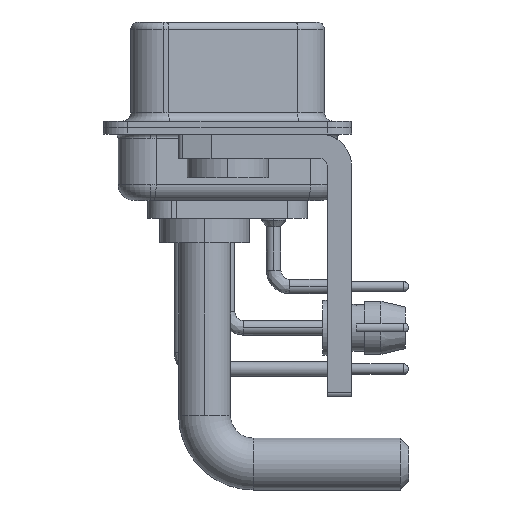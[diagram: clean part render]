
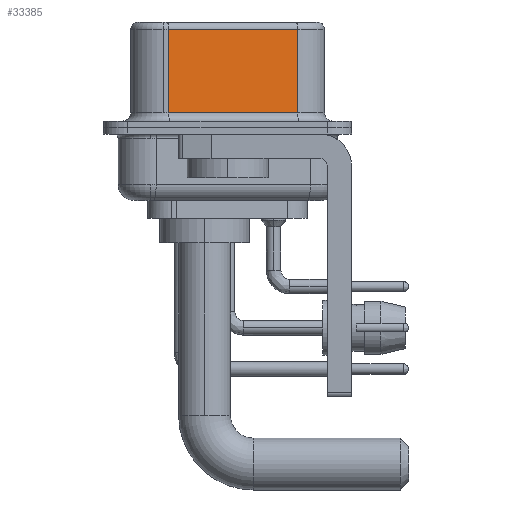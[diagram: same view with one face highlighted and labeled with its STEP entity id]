
A CAD part, left-side view. The second image highlights one B-rep face of the part: STEP entity #33385.
In plain terms, the highlighted planar face has unit normal (-0.985, -0.174, 0).
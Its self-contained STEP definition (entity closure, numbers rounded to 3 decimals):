
#1555 = CARTESIAN_POINT ( 'NONE',  ( 3.73, 3.628, 6.52 ) ) ;
#2030 = VECTOR ( 'NONE', #33905, 1000. ) ;
#3834 = VECTOR ( 'NONE', #34568, 1000. ) ;
#3892 = PLANE ( 'NONE',  #28740 ) ;
#5429 = VERTEX_POINT ( 'NONE', #19624 ) ;
#8009 = DIRECTION ( 'NONE',  ( -0.174, 0.985, 0. ) ) ;
#9073 = LINE ( 'NONE', #23927, #3834 ) ;
#9569 = CARTESIAN_POINT ( 'NONE',  ( 3.73, 3.628, 6.02 ) ) ;
#10023 = CARTESIAN_POINT ( 'NONE',  ( 5.132, -4.322, 6.52 ) ) ;
#13352 = EDGE_CURVE ( 'NONE', #21928, #5429, #9073, .T. ) ;
#14347 = LINE ( 'NONE', #24977, #2030 ) ;
#14448 = VERTEX_POINT ( 'NONE', #18462 ) ;
#14463 = VERTEX_POINT ( 'NONE', #9569 ) ;
#15104 = ORIENTED_EDGE ( 'NONE', *, *, #33988, .T. ) ;
#16024 = ORIENTED_EDGE ( 'NONE', *, *, #21166, .T. ) ;
#16779 = ORIENTED_EDGE ( 'NONE', *, *, #13352, .F. ) ;
#18462 = CARTESIAN_POINT ( 'NONE',  ( 3.73, 3.628, 0.9 ) ) ;
#19144 = LINE ( 'NONE', #33488, #27423 ) ;
#19624 = CARTESIAN_POINT ( 'NONE',  ( 5.132, -4.322, 0.9 ) ) ;
#21166 = EDGE_CURVE ( 'NONE', #21928, #14463, #19144, .T. ) ;
#21265 = LINE ( 'NONE', #1555, #33356 ) ;
#21466 = CARTESIAN_POINT ( 'NONE',  ( 5.132, -4.322, 6.02 ) ) ;
#21928 = VERTEX_POINT ( 'NONE', #21466 ) ;
#23927 = CARTESIAN_POINT ( 'NONE',  ( 5.132, -4.322, 6.52 ) ) ;
#24977 = CARTESIAN_POINT ( 'NONE',  ( 5.132, -4.322, 0.9 ) ) ;
#27423 = VECTOR ( 'NONE', #8009, 1000. ) ;
#28158 = EDGE_LOOP ( 'NONE', ( #16779, #16024, #33164, #15104 ) ) ;
#28740 = AXIS2_PLACEMENT_3D ( 'NONE', #10023, #35695, #35142 ) ;
#29550 = FACE_OUTER_BOUND ( 'NONE', #28158, .T. ) ;
#31376 = EDGE_CURVE ( 'NONE', #14463, #14448, #21265, .T. ) ;
#33164 = ORIENTED_EDGE ( 'NONE', *, *, #31376, .T. ) ;
#33176 = DIRECTION ( 'NONE',  ( 0., 0., -1. ) ) ;
#33356 = VECTOR ( 'NONE', #33176, 1000. ) ;
#33385 = ADVANCED_FACE ( 'NONE', ( #29550 ), #3892, .F. ) ;
#33488 = CARTESIAN_POINT ( 'NONE',  ( 5.132, -4.322, 6.02 ) ) ;
#33905 = DIRECTION ( 'NONE',  ( 0.174, -0.985, 0. ) ) ;
#33988 = EDGE_CURVE ( 'NONE', #14448, #5429, #14347, .T. ) ;
#34568 = DIRECTION ( 'NONE',  ( 0., 0., -1. ) ) ;
#35142 = DIRECTION ( 'NONE',  ( -0.174, 0.985, 0. ) ) ;
#35695 = DIRECTION ( 'NONE',  ( 0.985, 0.174, 0. ) ) ;
